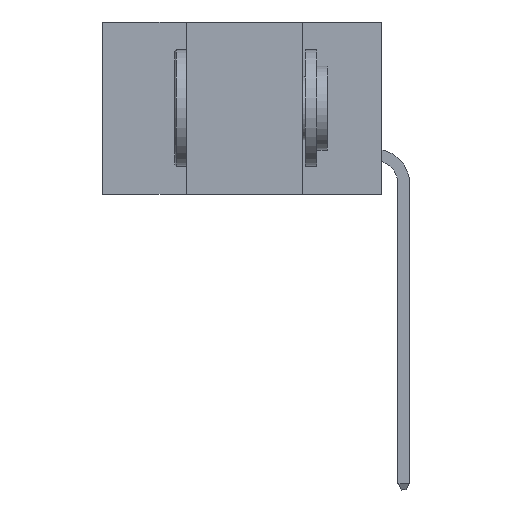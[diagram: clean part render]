
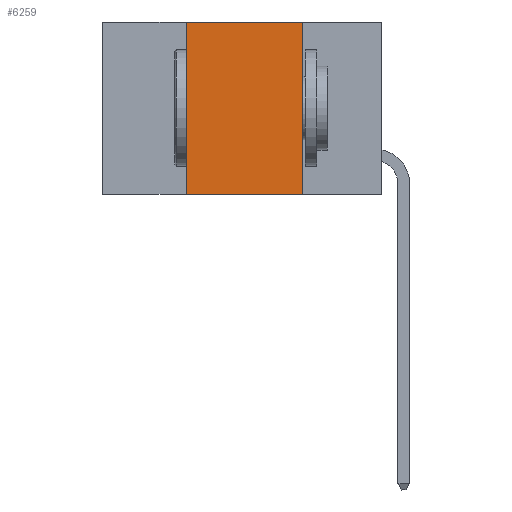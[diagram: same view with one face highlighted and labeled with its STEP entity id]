
A CAD part, left-side view. The second image highlights one B-rep face of the part: STEP entity #6259.
In plain terms, the highlighted planar face has unit normal (-1, 0, 0).
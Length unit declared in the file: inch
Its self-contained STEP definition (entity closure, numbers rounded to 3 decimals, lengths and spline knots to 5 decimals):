
#55 = VECTOR ( 'NONE', #5480, 39.37008 ) ;
#482 = VECTOR ( 'NONE', #3144, 39.37008 ) ;
#741 = CARTESIAN_POINT ( 'NONE',  ( 0., 0.6, 0. ) ) ;
#1182 = LINE ( 'NONE', #741, #3103 ) ;
#1556 = DIRECTION ( 'NONE',  ( 0., -1., 0. ) ) ;
#1730 = DIRECTION ( 'NONE',  ( 0., 0., -1. ) ) ;
#1771 = DIRECTION ( 'NONE',  ( 1., 0., 0. ) ) ;
#2234 = LINE ( 'NONE', #7425, #9510 ) ;
#2748 = PLANE ( 'NONE',  #5699 ) ;
#3023 = DIRECTION ( 'NONE',  ( 0., -1., 0. ) ) ;
#3103 = VECTOR ( 'NONE', #1556, 39.37008 ) ;
#3144 = DIRECTION ( 'NONE',  ( 0., 0., -1. ) ) ;
#3184 = CARTESIAN_POINT ( 'NONE',  ( 0., 0.17, 0. ) ) ;
#3192 = CARTESIAN_POINT ( 'NONE',  ( 0., 0.6, 0. ) ) ;
#3542 = VERTEX_POINT ( 'NONE', #7325 ) ;
#3919 = CARTESIAN_POINT ( 'NONE',  ( 0., 0.42, 0. ) ) ;
#4098 = VERTEX_POINT ( 'NONE', #3919 ) ;
#4111 = CARTESIAN_POINT ( 'NONE',  ( 0., 0.42, -0.37 ) ) ;
#4890 = FACE_OUTER_BOUND ( 'NONE', #5671, .T. ) ;
#5480 = DIRECTION ( 'NONE',  ( 0., 0., 1. ) ) ;
#5671 = EDGE_LOOP ( 'NONE', ( #7003, #7015, #7060, #7092 ) ) ;
#5699 = AXIS2_PLACEMENT_3D ( 'NONE', #3192, #1771, #1730 ) ;
#6259 = ADVANCED_FACE ( 'NONE', ( #4890 ), #2748, .F. ) ;
#6272 = LINE ( 'NONE', #7548, #55 ) ;
#6922 = EDGE_CURVE ( 'NONE', #3542, #7564, #8293, .T. ) ;
#7003 = ORIENTED_EDGE ( 'NONE', *, *, #6922, .F. ) ;
#7015 = ORIENTED_EDGE ( 'NONE', *, *, #8946, .F. ) ;
#7060 = ORIENTED_EDGE ( 'NONE', *, *, #9437, .F. ) ;
#7092 = ORIENTED_EDGE ( 'NONE', *, *, #7629, .T. ) ;
#7325 = CARTESIAN_POINT ( 'NONE',  ( 0., 0.17, 0. ) ) ;
#7425 = CARTESIAN_POINT ( 'NONE',  ( 0., 0.6, -0.37 ) ) ;
#7548 = CARTESIAN_POINT ( 'NONE',  ( 0., 0.42, 0. ) ) ;
#7564 = VERTEX_POINT ( 'NONE', #8085 ) ;
#7629 = EDGE_CURVE ( 'NONE', #9559, #7564, #2234, .T. ) ;
#8085 = CARTESIAN_POINT ( 'NONE',  ( 0., 0.17, -0.37 ) ) ;
#8293 = LINE ( 'NONE', #3184, #482 ) ;
#8946 = EDGE_CURVE ( 'NONE', #4098, #3542, #1182, .T. ) ;
#9437 = EDGE_CURVE ( 'NONE', #9559, #4098, #6272, .T. ) ;
#9510 = VECTOR ( 'NONE', #3023, 39.37008 ) ;
#9559 = VERTEX_POINT ( 'NONE', #4111 ) ;
